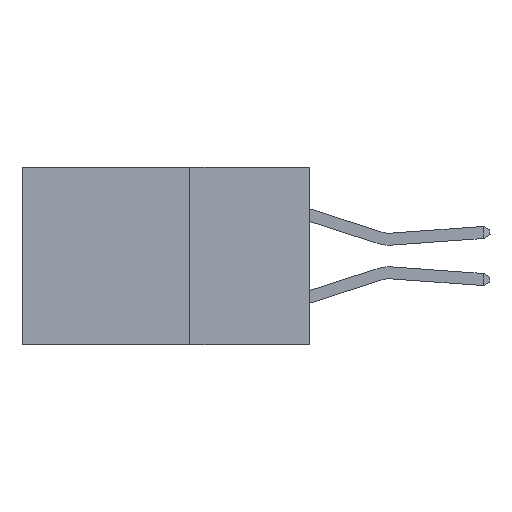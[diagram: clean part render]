
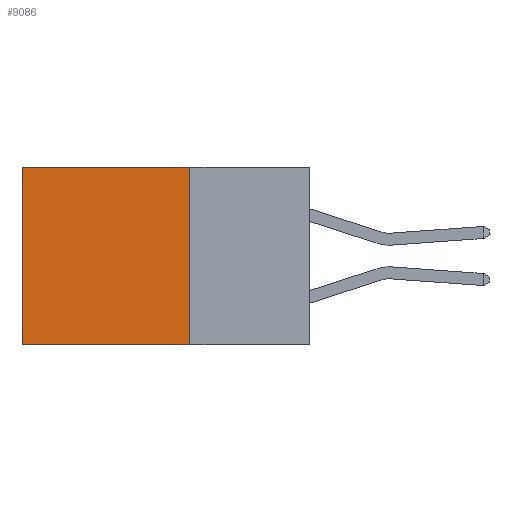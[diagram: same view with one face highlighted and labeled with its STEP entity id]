
A CAD part, left-side view. The second image highlights one B-rep face of the part: STEP entity #9086.
In plain terms, the highlighted planar face has unit normal (-1, 0, 0).
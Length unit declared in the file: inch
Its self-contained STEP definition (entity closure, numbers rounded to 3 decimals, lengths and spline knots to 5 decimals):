
#260 = CARTESIAN_POINT ( 'NONE',  ( 0.2615, 0.25, 0. ) ) ;
#696 = EDGE_CURVE ( 'NONE', #7503, #9067, #1223, .T. ) ;
#907 = VECTOR ( 'NONE', #7645, 39.37008 ) ;
#1223 = LINE ( 'NONE', #9008, #907 ) ;
#1326 = VERTEX_POINT ( 'NONE', #260 ) ;
#1467 = ORIENTED_EDGE ( 'NONE', *, *, #8072, .T. ) ;
#1838 = CARTESIAN_POINT ( 'NONE',  ( 0.2615, 0.6, -0.37 ) ) ;
#2605 = ORIENTED_EDGE ( 'NONE', *, *, #4618, .T. ) ;
#2654 = ORIENTED_EDGE ( 'NONE', *, *, #696, .F. ) ;
#3028 = VECTOR ( 'NONE', #7205, 39.37008 ) ;
#3823 = AXIS2_PLACEMENT_3D ( 'NONE', #3921, #8286, #6831 ) ;
#3921 = CARTESIAN_POINT ( 'NONE',  ( 0.2615, 0.25, -0.37 ) ) ;
#4021 = PLANE ( 'NONE',  #3823 ) ;
#4416 = LINE ( 'NONE', #8762, #3028 ) ;
#4466 = DIRECTION ( 'NONE',  ( 0., 1., 0. ) ) ;
#4511 = DIRECTION ( 'NONE',  ( 0., 0., -1. ) ) ;
#4618 = EDGE_CURVE ( 'NONE', #1326, #5352, #8583, .T. ) ;
#4950 = VECTOR ( 'NONE', #4466, 39.37008 ) ;
#5324 = FACE_OUTER_BOUND ( 'NONE', #8409, .T. ) ;
#5352 = VERTEX_POINT ( 'NONE', #5750 ) ;
#5451 = VECTOR ( 'NONE', #4511, 39.37008 ) ;
#5591 = EDGE_CURVE ( 'NONE', #1326, #7503, #4416, .T. ) ;
#5750 = CARTESIAN_POINT ( 'NONE',  ( 0.2615, 0.6, 0. ) ) ;
#6182 = CARTESIAN_POINT ( 'NONE',  ( 0.2615, 0.25, -0.37 ) ) ;
#6626 = CARTESIAN_POINT ( 'NONE',  ( 0.2615, 0.25, 0. ) ) ;
#6831 = DIRECTION ( 'NONE',  ( 0., 0., -1. ) ) ;
#7205 = DIRECTION ( 'NONE',  ( 0., 0., -1. ) ) ;
#7451 = LINE ( 'NONE', #7982, #5451 ) ;
#7503 = VERTEX_POINT ( 'NONE', #6182 ) ;
#7645 = DIRECTION ( 'NONE',  ( 0., 1., 0. ) ) ;
#7982 = CARTESIAN_POINT ( 'NONE',  ( 0.2615, 0.6, -0.37 ) ) ;
#8072 = EDGE_CURVE ( 'NONE', #5352, #9067, #7451, .T. ) ;
#8286 = DIRECTION ( 'NONE',  ( 1., 0., 0. ) ) ;
#8409 = EDGE_LOOP ( 'NONE', ( #1467, #2654, #8575, #2605 ) ) ;
#8575 = ORIENTED_EDGE ( 'NONE', *, *, #5591, .F. ) ;
#8583 = LINE ( 'NONE', #6626, #4950 ) ;
#8762 = CARTESIAN_POINT ( 'NONE',  ( 0.2615, 0.25, -0.37 ) ) ;
#9008 = CARTESIAN_POINT ( 'NONE',  ( 0.2615, 0.25, -0.37 ) ) ;
#9067 = VERTEX_POINT ( 'NONE', #1838 ) ;
#9086 = ADVANCED_FACE ( 'NONE', ( #5324 ), #4021, .F. ) ;
